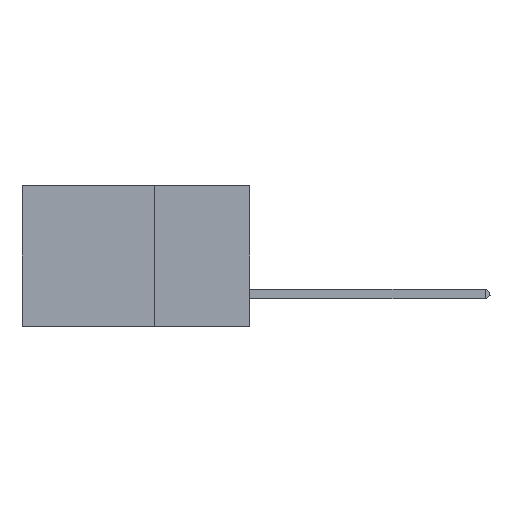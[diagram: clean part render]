
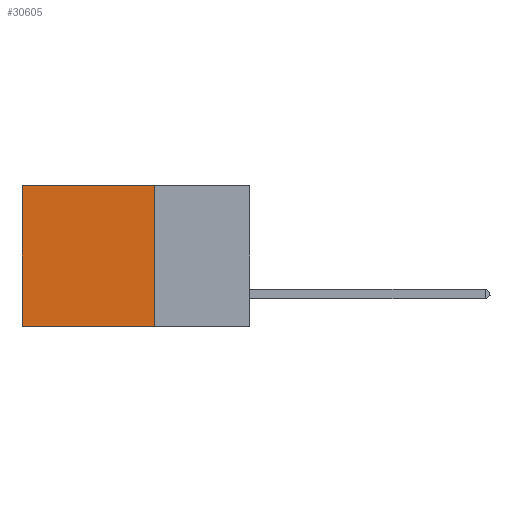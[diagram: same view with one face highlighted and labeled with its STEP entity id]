
A CAD part, left-side view. The second image highlights one B-rep face of the part: STEP entity #30605.
In plain terms, the highlighted planar face has unit normal (-1, 0, 0).
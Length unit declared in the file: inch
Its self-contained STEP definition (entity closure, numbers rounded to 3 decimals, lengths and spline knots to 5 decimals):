
#81 = VECTOR ( 'NONE', #11662, 39.37008 ) ;
#281 = PLANE ( 'NONE',  #27019 ) ;
#1580 = LINE ( 'NONE', #16897, #9929 ) ;
#1984 = EDGE_CURVE ( 'NONE', #23187, #8037, #4418, .T. ) ;
#3030 = EDGE_LOOP ( 'NONE', ( #23836, #6252, #20078, #6230 ) ) ;
#3879 = EDGE_CURVE ( 'NONE', #23187, #10160, #1580, .T. ) ;
#4418 = LINE ( 'NONE', #27358, #81 ) ;
#5605 = VECTOR ( 'NONE', #23716, 39.37008 ) ;
#5649 = FACE_OUTER_BOUND ( 'NONE', #3030, .T. ) ;
#6230 = ORIENTED_EDGE ( 'NONE', *, *, #1984, .T. ) ;
#6252 = ORIENTED_EDGE ( 'NONE', *, *, #18432, .F. ) ;
#7529 = CARTESIAN_POINT ( 'NONE',  ( 0.2875, 0.25, 0. ) ) ;
#8013 = DIRECTION ( 'NONE',  ( 1., 0., 0. ) ) ;
#8037 = VERTEX_POINT ( 'NONE', #11743 ) ;
#9122 = VECTOR ( 'NONE', #33102, 39.37008 ) ;
#9929 = VECTOR ( 'NONE', #32914, 39.37008 ) ;
#10160 = VERTEX_POINT ( 'NONE', #32984 ) ;
#11662 = DIRECTION ( 'NONE',  ( 0., 1., 0. ) ) ;
#11743 = CARTESIAN_POINT ( 'NONE',  ( 0.2875, 0.6, 0. ) ) ;
#12371 = LINE ( 'NONE', #19965, #9122 ) ;
#13430 = CARTESIAN_POINT ( 'NONE',  ( 0.2875, 0.25, -0.37 ) ) ;
#16897 = CARTESIAN_POINT ( 'NONE',  ( 0.2875, 0.25, 0. ) ) ;
#17979 = DIRECTION ( 'NONE',  ( 0., 0., -1. ) ) ;
#18432 = EDGE_CURVE ( 'NONE', #10160, #19326, #28616, .T. ) ;
#19326 = VERTEX_POINT ( 'NONE', #25682 ) ;
#19965 = CARTESIAN_POINT ( 'NONE',  ( 0.2875, 0.6, 0. ) ) ;
#20078 = ORIENTED_EDGE ( 'NONE', *, *, #3879, .F. ) ;
#23187 = VERTEX_POINT ( 'NONE', #26497 ) ;
#23716 = DIRECTION ( 'NONE',  ( 0., 1., 0. ) ) ;
#23836 = ORIENTED_EDGE ( 'NONE', *, *, #24443, .T. ) ;
#24443 = EDGE_CURVE ( 'NONE', #8037, #19326, #12371, .T. ) ;
#25682 = CARTESIAN_POINT ( 'NONE',  ( 0.2875, 0.6, -0.37 ) ) ;
#26497 = CARTESIAN_POINT ( 'NONE',  ( 0.2875, 0.25, 0. ) ) ;
#27019 = AXIS2_PLACEMENT_3D ( 'NONE', #7529, #8013, #17979 ) ;
#27358 = CARTESIAN_POINT ( 'NONE',  ( 0.2875, 0.25, 0. ) ) ;
#28616 = LINE ( 'NONE', #13430, #5605 ) ;
#30605 = ADVANCED_FACE ( 'NONE', ( #5649 ), #281, .F. ) ;
#32914 = DIRECTION ( 'NONE',  ( 0., 0., -1. ) ) ;
#32984 = CARTESIAN_POINT ( 'NONE',  ( 0.2875, 0.25, -0.37 ) ) ;
#33102 = DIRECTION ( 'NONE',  ( 0., 0., -1. ) ) ;
